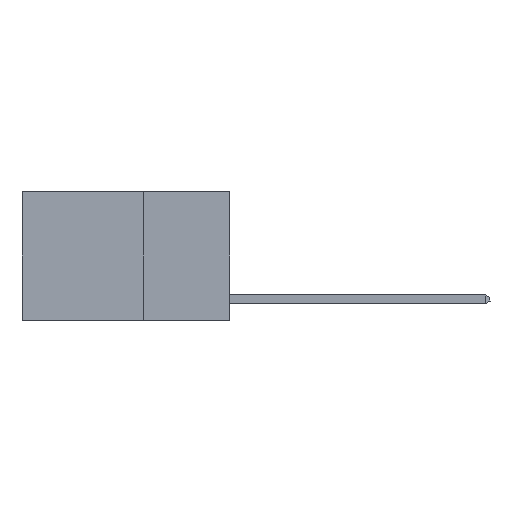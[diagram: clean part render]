
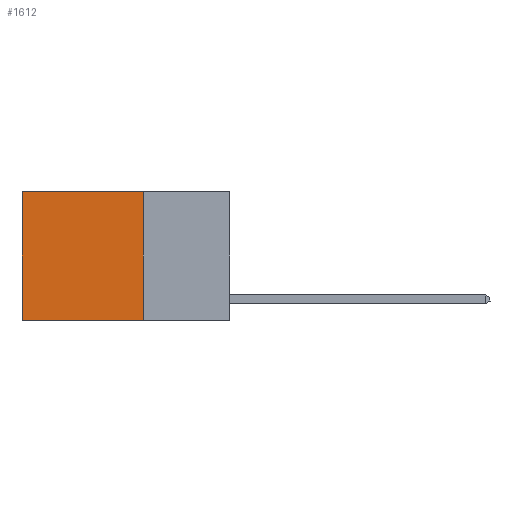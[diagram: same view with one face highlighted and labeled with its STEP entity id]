
A CAD part, left-side view. The second image highlights one B-rep face of the part: STEP entity #1612.
In plain terms, the highlighted planar face has unit normal (-1, 0, 0).
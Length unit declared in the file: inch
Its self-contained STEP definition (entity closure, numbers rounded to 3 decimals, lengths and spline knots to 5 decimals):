
#243 = EDGE_LOOP ( 'NONE', ( #7231, #4403, #1515, #9197 ) ) ;
#281 = LINE ( 'NONE', #7762, #10646 ) ;
#312 = EDGE_CURVE ( 'NONE', #10954, #2507, #281, .T. ) ;
#380 = DIRECTION ( 'NONE',  ( 0., 0., -1. ) ) ;
#1384 = EDGE_CURVE ( 'NONE', #3502, #2507, #8548, .T. ) ;
#1515 = ORIENTED_EDGE ( 'NONE', *, *, #11293, .F. ) ;
#1612 = ADVANCED_FACE ( 'NONE', ( #3389 ), #8120, .F. ) ;
#1664 = LINE ( 'NONE', #2365, #12010 ) ;
#2365 = CARTESIAN_POINT ( 'NONE',  ( 0.2625, 0.25, 0. ) ) ;
#2507 = VERTEX_POINT ( 'NONE', #12836 ) ;
#2801 = CARTESIAN_POINT ( 'NONE',  ( 0.2625, 0.6, 0. ) ) ;
#3389 = FACE_OUTER_BOUND ( 'NONE', #243, .T. ) ;
#3502 = VERTEX_POINT ( 'NONE', #8632 ) ;
#3821 = DIRECTION ( 'NONE',  ( 0., 1., 0. ) ) ;
#4403 = ORIENTED_EDGE ( 'NONE', *, *, #1384, .F. ) ;
#4655 = DIRECTION ( 'NONE',  ( 0., 0., -1. ) ) ;
#5161 = VECTOR ( 'NONE', #11398, 39.37008 ) ;
#5688 = CARTESIAN_POINT ( 'NONE',  ( 0.2625, 0.25, 0. ) ) ;
#6572 = VECTOR ( 'NONE', #3821, 39.37008 ) ;
#7231 = ORIENTED_EDGE ( 'NONE', *, *, #312, .T. ) ;
#7762 = CARTESIAN_POINT ( 'NONE',  ( 0.2625, 0.6, 0. ) ) ;
#7998 = DIRECTION ( 'NONE',  ( 0., 0., -1. ) ) ;
#8059 = DIRECTION ( 'NONE',  ( 1., 0., 0. ) ) ;
#8120 = PLANE ( 'NONE',  #12670 ) ;
#8190 = CARTESIAN_POINT ( 'NONE',  ( 0.2625, 0.25, 0. ) ) ;
#8548 = LINE ( 'NONE', #11894, #5161 ) ;
#8632 = CARTESIAN_POINT ( 'NONE',  ( 0.2625, 0.25, -0.37 ) ) ;
#9197 = ORIENTED_EDGE ( 'NONE', *, *, #10982, .T. ) ;
#9395 = LINE ( 'NONE', #5688, #6572 ) ;
#10646 = VECTOR ( 'NONE', #4655, 39.37008 ) ;
#10954 = VERTEX_POINT ( 'NONE', #2801 ) ;
#10982 = EDGE_CURVE ( 'NONE', #12260, #10954, #9395, .T. ) ;
#11293 = EDGE_CURVE ( 'NONE', #12260, #3502, #1664, .T. ) ;
#11354 = CARTESIAN_POINT ( 'NONE',  ( 0.2625, 0.25, 0. ) ) ;
#11398 = DIRECTION ( 'NONE',  ( 0., 1., 0. ) ) ;
#11894 = CARTESIAN_POINT ( 'NONE',  ( 0.2625, 0.25, -0.37 ) ) ;
#12010 = VECTOR ( 'NONE', #380, 39.37008 ) ;
#12260 = VERTEX_POINT ( 'NONE', #11354 ) ;
#12670 = AXIS2_PLACEMENT_3D ( 'NONE', #8190, #8059, #7998 ) ;
#12836 = CARTESIAN_POINT ( 'NONE',  ( 0.2625, 0.6, -0.37 ) ) ;
